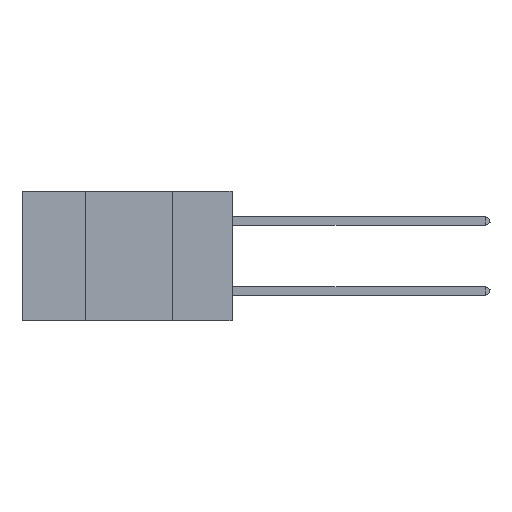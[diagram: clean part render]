
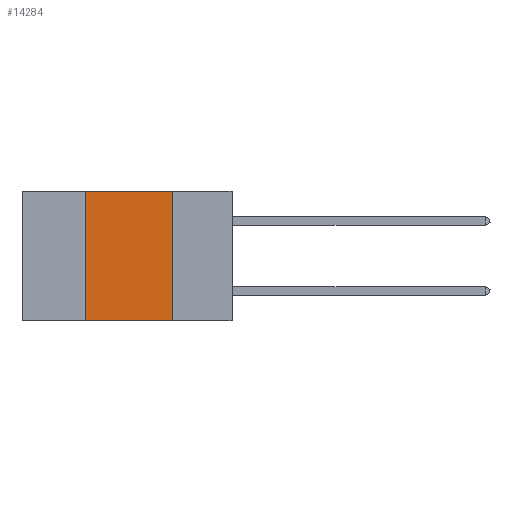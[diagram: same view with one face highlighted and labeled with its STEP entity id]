
A CAD part, left-side view. The second image highlights one B-rep face of the part: STEP entity #14284.
In plain terms, the highlighted planar face has unit normal (-1, 0, 0).
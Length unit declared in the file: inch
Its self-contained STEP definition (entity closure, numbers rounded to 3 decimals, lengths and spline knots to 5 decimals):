
#52 = ORIENTED_EDGE ( 'NONE', *, *, #25499, .F. ) ;
#2707 = VECTOR ( 'NONE', #12373, 39.37008 ) ;
#2744 = DIRECTION ( 'NONE',  ( 0., 0., 1. ) ) ;
#5821 = ORIENTED_EDGE ( 'NONE', *, *, #17592, .F. ) ;
#6280 = CARTESIAN_POINT ( 'NONE',  ( 0., 0.42, 0. ) ) ;
#8211 = CARTESIAN_POINT ( 'NONE',  ( 0., 0.17, 0. ) ) ;
#8934 = DIRECTION ( 'NONE',  ( 0., -1., 0. ) ) ;
#9374 = VECTOR ( 'NONE', #31928, 39.37008 ) ;
#9490 = VERTEX_POINT ( 'NONE', #25291 ) ;
#11735 = LINE ( 'NONE', #8211, #9374 ) ;
#12109 = CARTESIAN_POINT ( 'NONE',  ( 0., 0.6, 0. ) ) ;
#12373 = DIRECTION ( 'NONE',  ( 0., -1., 0. ) ) ;
#12947 = VERTEX_POINT ( 'NONE', #6280 ) ;
#13196 = VERTEX_POINT ( 'NONE', #31670 ) ;
#14284 = ADVANCED_FACE ( 'NONE', ( #29233 ), #15487, .F. ) ;
#14429 = LINE ( 'NONE', #12109, #2707 ) ;
#15487 = PLANE ( 'NONE',  #36737 ) ;
#16018 = EDGE_CURVE ( 'NONE', #9490, #24300, #11735, .T. ) ;
#17592 = EDGE_CURVE ( 'NONE', #13196, #12947, #38265, .T. ) ;
#19044 = ORIENTED_EDGE ( 'NONE', *, *, #16018, .F. ) ;
#20008 = VECTOR ( 'NONE', #8934, 39.37008 ) ;
#20284 = CARTESIAN_POINT ( 'NONE',  ( 0., 0.42, 0. ) ) ;
#20852 = CARTESIAN_POINT ( 'NONE',  ( 0., 0.6, -0.37 ) ) ;
#21460 = LINE ( 'NONE', #20852, #20008 ) ;
#24300 = VERTEX_POINT ( 'NONE', #33009 ) ;
#24791 = CARTESIAN_POINT ( 'NONE',  ( 0., 0.6, 0. ) ) ;
#25291 = CARTESIAN_POINT ( 'NONE',  ( 0., 0.17, 0. ) ) ;
#25499 = EDGE_CURVE ( 'NONE', #12947, #9490, #14429, .T. ) ;
#26853 = EDGE_CURVE ( 'NONE', #13196, #24300, #21460, .T. ) ;
#27924 = DIRECTION ( 'NONE',  ( 1., 0., 0. ) ) ;
#28471 = VECTOR ( 'NONE', #2744, 39.37008 ) ;
#29150 = ORIENTED_EDGE ( 'NONE', *, *, #26853, .T. ) ;
#29233 = FACE_OUTER_BOUND ( 'NONE', #33737, .T. ) ;
#30682 = DIRECTION ( 'NONE',  ( 0., 0., -1. ) ) ;
#31670 = CARTESIAN_POINT ( 'NONE',  ( 0., 0.42, -0.37 ) ) ;
#31928 = DIRECTION ( 'NONE',  ( 0., 0., -1. ) ) ;
#33009 = CARTESIAN_POINT ( 'NONE',  ( 0., 0.17, -0.37 ) ) ;
#33737 = EDGE_LOOP ( 'NONE', ( #19044, #52, #5821, #29150 ) ) ;
#36737 = AXIS2_PLACEMENT_3D ( 'NONE', #24791, #27924, #30682 ) ;
#38265 = LINE ( 'NONE', #20284, #28471 ) ;
